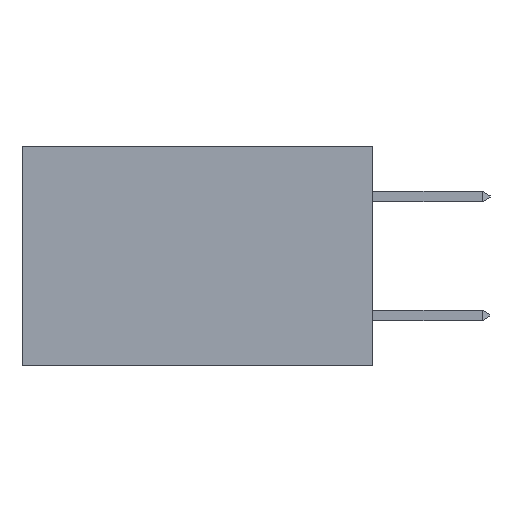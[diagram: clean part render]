
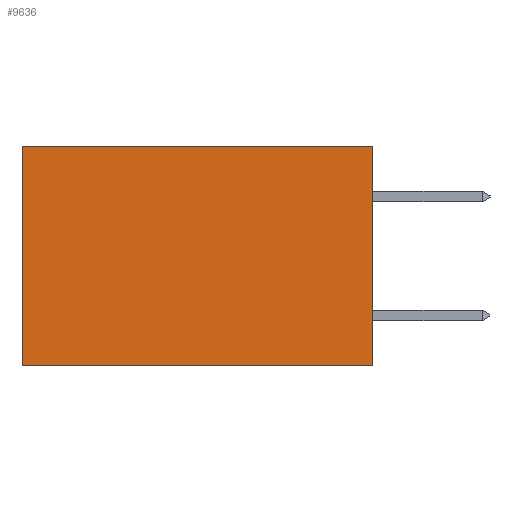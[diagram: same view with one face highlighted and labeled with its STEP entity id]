
A CAD part, left-side view. The second image highlights one B-rep face of the part: STEP entity #9636.
In plain terms, the highlighted planar face has unit normal (-1, 0, 0).
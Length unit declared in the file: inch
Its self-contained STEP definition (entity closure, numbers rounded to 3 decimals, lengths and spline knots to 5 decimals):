
#165 = DIRECTION ( 'NONE',  ( 0., 1., 0. ) ) ;
#178 = ORIENTED_EDGE ( 'NONE', *, *, #1980, .F. ) ;
#1980 = EDGE_CURVE ( 'NONE', #8139, #24353, #5457, .T. ) ;
#3322 = EDGE_CURVE ( 'NONE', #24353, #20169, #10165, .T. ) ;
#3750 = EDGE_CURVE ( 'NONE', #8139, #11837, #17344, .T. ) ;
#5457 = LINE ( 'NONE', #21524, #28176 ) ;
#6241 = VECTOR ( 'NONE', #29995, 39.37008 ) ;
#6389 = AXIS2_PLACEMENT_3D ( 'NONE', #22195, #24651, #10113 ) ;
#8139 = VERTEX_POINT ( 'NONE', #26776 ) ;
#9453 = CARTESIAN_POINT ( 'NONE',  ( 0.277, 0., -0.37 ) ) ;
#9636 = ADVANCED_FACE ( 'NONE', ( #31067 ), #19740, .F. ) ;
#10055 = CARTESIAN_POINT ( 'NONE',  ( 0.277, 0.59, -0.37 ) ) ;
#10113 = DIRECTION ( 'NONE',  ( 0., 0., -1. ) ) ;
#10165 = LINE ( 'NONE', #27133, #23078 ) ;
#10278 = CARTESIAN_POINT ( 'NONE',  ( 0.277, 0.59, 0. ) ) ;
#10875 = VECTOR ( 'NONE', #28299, 39.37008 ) ;
#11837 = VERTEX_POINT ( 'NONE', #10278 ) ;
#11883 = LINE ( 'NONE', #22634, #6241 ) ;
#12620 = EDGE_CURVE ( 'NONE', #11837, #20169, #11883, .T. ) ;
#16666 = ORIENTED_EDGE ( 'NONE', *, *, #3322, .F. ) ;
#17344 = LINE ( 'NONE', #29399, #10875 ) ;
#17990 = DIRECTION ( 'NONE',  ( 0., 0., -1. ) ) ;
#18918 = ORIENTED_EDGE ( 'NONE', *, *, #12620, .T. ) ;
#19740 = PLANE ( 'NONE',  #6389 ) ;
#20169 = VERTEX_POINT ( 'NONE', #10055 ) ;
#21524 = CARTESIAN_POINT ( 'NONE',  ( 0.277, 0., -0.37 ) ) ;
#22195 = CARTESIAN_POINT ( 'NONE',  ( 0.277, 0., -0.37 ) ) ;
#22634 = CARTESIAN_POINT ( 'NONE',  ( 0.277, 0.59, -0.37 ) ) ;
#23078 = VECTOR ( 'NONE', #165, 39.37008 ) ;
#23448 = EDGE_LOOP ( 'NONE', ( #18918, #16666, #178, #23704 ) ) ;
#23704 = ORIENTED_EDGE ( 'NONE', *, *, #3750, .T. ) ;
#24353 = VERTEX_POINT ( 'NONE', #9453 ) ;
#24651 = DIRECTION ( 'NONE',  ( 1., 0., 0. ) ) ;
#26776 = CARTESIAN_POINT ( 'NONE',  ( 0.277, 0., 0. ) ) ;
#27133 = CARTESIAN_POINT ( 'NONE',  ( 0.277, 0., -0.37 ) ) ;
#28176 = VECTOR ( 'NONE', #17990, 39.37008 ) ;
#28299 = DIRECTION ( 'NONE',  ( 0., 1., 0. ) ) ;
#29399 = CARTESIAN_POINT ( 'NONE',  ( 0.277, 0., 0. ) ) ;
#29995 = DIRECTION ( 'NONE',  ( 0., 0., -1. ) ) ;
#31067 = FACE_OUTER_BOUND ( 'NONE', #23448, .T. ) ;
